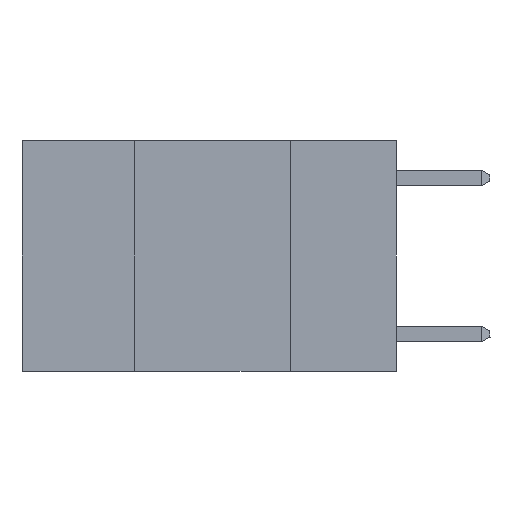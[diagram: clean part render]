
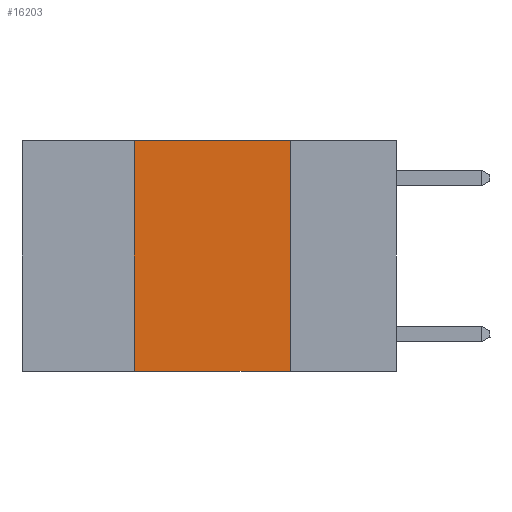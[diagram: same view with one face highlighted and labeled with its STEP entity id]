
A CAD part, left-side view. The second image highlights one B-rep face of the part: STEP entity #16203.
In plain terms, the highlighted planar face has unit normal (-1, 0, 0).
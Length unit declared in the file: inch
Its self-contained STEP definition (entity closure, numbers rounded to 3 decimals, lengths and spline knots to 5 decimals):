
#254 = AXIS2_PLACEMENT_3D ( 'NONE', #10649, #15636, #1941 ) ;
#475 = DIRECTION ( 'NONE',  ( 0., 0., 1. ) ) ;
#909 = LINE ( 'NONE', #11512, #17848 ) ;
#1473 = CARTESIAN_POINT ( 'NONE',  ( 0., 0.17, -0.37 ) ) ;
#1542 = FACE_OUTER_BOUND ( 'NONE', #5031, .T. ) ;
#1941 = DIRECTION ( 'NONE',  ( 0., 0., -1. ) ) ;
#2440 = VECTOR ( 'NONE', #10976, 39.37008 ) ;
#3070 = LINE ( 'NONE', #4649, #2440 ) ;
#4232 = EDGE_CURVE ( 'NONE', #14834, #19533, #909, .T. ) ;
#4340 = ORIENTED_EDGE ( 'NONE', *, *, #11306, .T. ) ;
#4649 = CARTESIAN_POINT ( 'NONE',  ( 0., 0.6, -0.37 ) ) ;
#4990 = VERTEX_POINT ( 'NONE', #8033 ) ;
#5031 = EDGE_LOOP ( 'NONE', ( #19418, #11231, #6917, #4340 ) ) ;
#5294 = VECTOR ( 'NONE', #15086, 39.37008 ) ;
#5874 = LINE ( 'NONE', #10301, #5294 ) ;
#6917 = ORIENTED_EDGE ( 'NONE', *, *, #8102, .F. ) ;
#6937 = CARTESIAN_POINT ( 'NONE',  ( 0., 0.42, 0. ) ) ;
#8033 = CARTESIAN_POINT ( 'NONE',  ( 0., 0.42, -0.37 ) ) ;
#8102 = EDGE_CURVE ( 'NONE', #4990, #14834, #17122, .T. ) ;
#8187 = DIRECTION ( 'NONE',  ( 0., -1., 0. ) ) ;
#10301 = CARTESIAN_POINT ( 'NONE',  ( 0., 0.17, 0. ) ) ;
#10649 = CARTESIAN_POINT ( 'NONE',  ( 0., 0.6, 0. ) ) ;
#10682 = EDGE_CURVE ( 'NONE', #19533, #15935, #5874, .T. ) ;
#10976 = DIRECTION ( 'NONE',  ( 0., -1., 0. ) ) ;
#11181 = VECTOR ( 'NONE', #475, 39.37008 ) ;
#11231 = ORIENTED_EDGE ( 'NONE', *, *, #4232, .F. ) ;
#11306 = EDGE_CURVE ( 'NONE', #4990, #15935, #3070, .T. ) ;
#11512 = CARTESIAN_POINT ( 'NONE',  ( 0., 0.6, 0. ) ) ;
#13761 = PLANE ( 'NONE',  #254 ) ;
#14423 = CARTESIAN_POINT ( 'NONE',  ( 0., 0.17, 0. ) ) ;
#14834 = VERTEX_POINT ( 'NONE', #6937 ) ;
#15086 = DIRECTION ( 'NONE',  ( 0., 0., -1. ) ) ;
#15460 = CARTESIAN_POINT ( 'NONE',  ( 0., 0.42, 0. ) ) ;
#15636 = DIRECTION ( 'NONE',  ( 1., 0., 0. ) ) ;
#15935 = VERTEX_POINT ( 'NONE', #1473 ) ;
#16203 = ADVANCED_FACE ( 'NONE', ( #1542 ), #13761, .F. ) ;
#17122 = LINE ( 'NONE', #15460, #11181 ) ;
#17848 = VECTOR ( 'NONE', #8187, 39.37008 ) ;
#19418 = ORIENTED_EDGE ( 'NONE', *, *, #10682, .F. ) ;
#19533 = VERTEX_POINT ( 'NONE', #14423 ) ;
